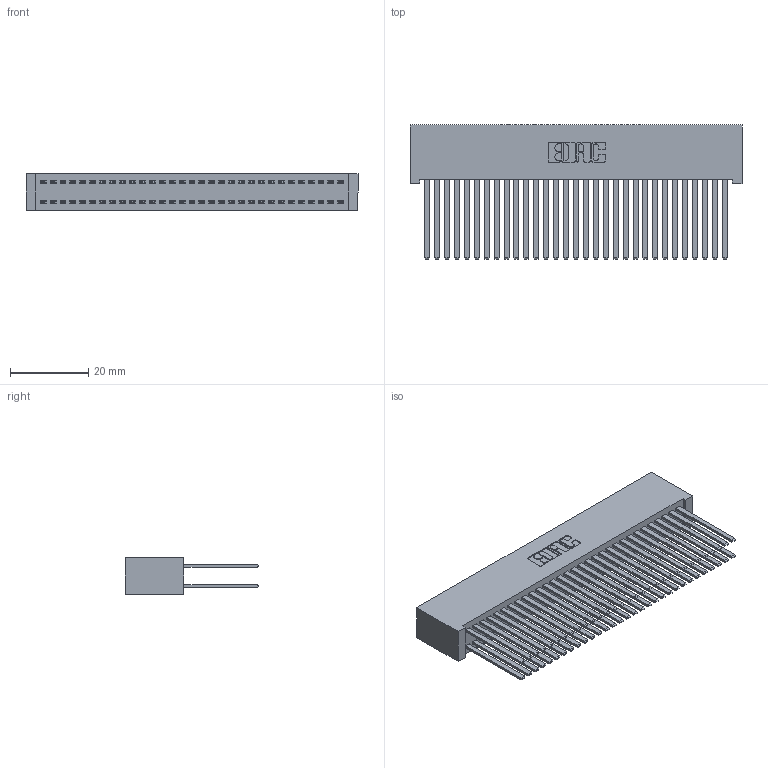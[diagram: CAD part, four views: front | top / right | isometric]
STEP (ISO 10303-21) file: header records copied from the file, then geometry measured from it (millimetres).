
FILE_DESCRIPTION (( 'STEP AP203' ), '1' );
FILE_NAME ('392-062-544-201.STEP', '2018-08-17T21:11:21', ( '' ), ( '' ), 'SwSTEP 2.0', 'SolidWorks 2016', '' );
FILE_SCHEMA (( 'CONFIG_CONTROL_DESIGN' ));
Length unit declared in the file: inch
Products named in the file (3): 342 Part_Lugless; 345-292-001_345-293-144; 392-062-544-201
Assembly tree (63 placements, depth 2):
  392-062-544-201
    342 Part_Lugless
    345-292-001_345-293-144  x62
Bounding box: 84.99 x 34.3 x 9.4 mm (x, y, z)
Volume: 8892.8 mm3; surface area: 17057.3 mm2
Topology: 63 solids, 63 shells, 2954 faces, 8769 edges, 5762 vertices
Faces by surface type: plane 2046, cylinder 908
Entity records: 20773 total; most frequent: CARTESIAN_POINT 3450, ORIENTED_EDGE 3386, DIRECTION 2957, EDGE_CURVE 1693, VECTOR 1577, LINE 1577, VERTEX_POINT 1126, AXIS2_PLACEMENT_3D 690
